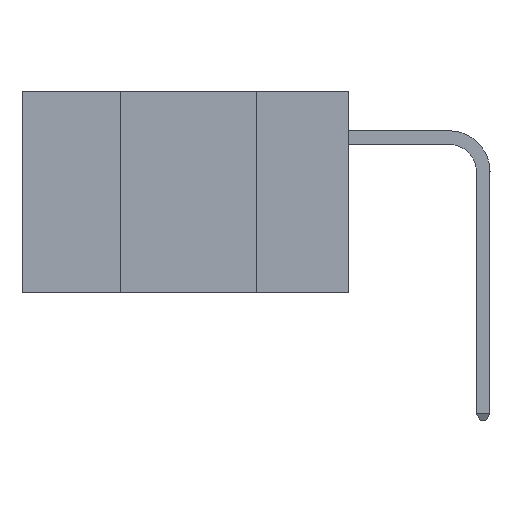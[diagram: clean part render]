
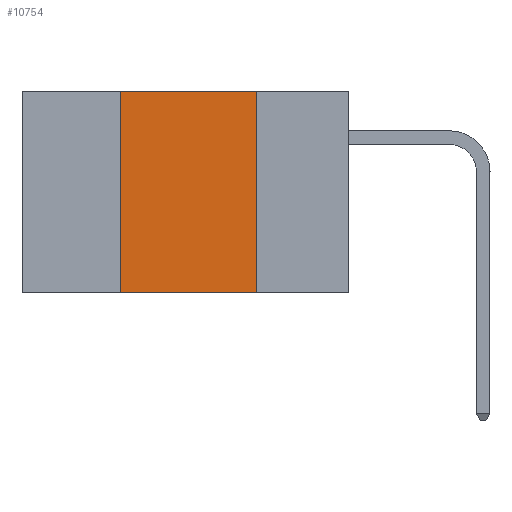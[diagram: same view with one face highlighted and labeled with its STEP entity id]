
A CAD part, left-side view. The second image highlights one B-rep face of the part: STEP entity #10754.
In plain terms, the highlighted planar face has unit normal (-1, 0, 0).
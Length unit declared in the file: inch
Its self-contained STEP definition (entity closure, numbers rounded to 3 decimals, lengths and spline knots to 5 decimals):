
#1278 = LINE ( 'NONE', #29180, #15102 ) ;
#1377 = AXIS2_PLACEMENT_3D ( 'NONE', #20924, #40406, #5973 ) ;
#1792 = EDGE_CURVE ( 'NONE', #21485, #6824, #11633, .T. ) ;
#2624 = DIRECTION ( 'NONE',  ( 0., 0., -1. ) ) ;
#2697 = EDGE_CURVE ( 'NONE', #21485, #25090, #6118, .T. ) ;
#4278 = LINE ( 'NONE', #31391, #24655 ) ;
#5049 = ORIENTED_EDGE ( 'NONE', *, *, #48254, .F. ) ;
#5973 = DIRECTION ( 'NONE',  ( 0., 0., -1. ) ) ;
#6118 = LINE ( 'NONE', #34220, #27786 ) ;
#6824 = VERTEX_POINT ( 'NONE', #37957 ) ;
#10754 = ADVANCED_FACE ( 'NONE', ( #14118 ), #32382, .F. ) ;
#11633 = LINE ( 'NONE', #17485, #30293 ) ;
#12376 = EDGE_CURVE ( 'NONE', #15441, #6824, #1278, .T. ) ;
#13359 = DIRECTION ( 'NONE',  ( 0., -1., 0. ) ) ;
#13405 = CARTESIAN_POINT ( 'NONE',  ( 0., 0.42, 0. ) ) ;
#13612 = DIRECTION ( 'NONE',  ( 0., -1., 0. ) ) ;
#14118 = FACE_OUTER_BOUND ( 'NONE', #40738, .T. ) ;
#15102 = VECTOR ( 'NONE', #2624, 39.37008 ) ;
#15112 = ORIENTED_EDGE ( 'NONE', *, *, #1792, .T. ) ;
#15441 = VERTEX_POINT ( 'NONE', #28796 ) ;
#16535 = ORIENTED_EDGE ( 'NONE', *, *, #12376, .F. ) ;
#17485 = CARTESIAN_POINT ( 'NONE',  ( 0., 0.6, -0.37 ) ) ;
#20924 = CARTESIAN_POINT ( 'NONE',  ( 0., 0.6, 0. ) ) ;
#21485 = VERTEX_POINT ( 'NONE', #27293 ) ;
#22627 = DIRECTION ( 'NONE',  ( 0., 0., 1. ) ) ;
#24655 = VECTOR ( 'NONE', #13359, 39.37008 ) ;
#25090 = VERTEX_POINT ( 'NONE', #13405 ) ;
#27293 = CARTESIAN_POINT ( 'NONE',  ( 0., 0.42, -0.37 ) ) ;
#27786 = VECTOR ( 'NONE', #22627, 39.37008 ) ;
#28721 = ORIENTED_EDGE ( 'NONE', *, *, #2697, .F. ) ;
#28796 = CARTESIAN_POINT ( 'NONE',  ( 0., 0.17, 0. ) ) ;
#29180 = CARTESIAN_POINT ( 'NONE',  ( 0., 0.17, 0. ) ) ;
#30293 = VECTOR ( 'NONE', #13612, 39.37008 ) ;
#31391 = CARTESIAN_POINT ( 'NONE',  ( 0., 0.6, 0. ) ) ;
#32382 = PLANE ( 'NONE',  #1377 ) ;
#34220 = CARTESIAN_POINT ( 'NONE',  ( 0., 0.42, 0. ) ) ;
#37957 = CARTESIAN_POINT ( 'NONE',  ( 0., 0.17, -0.37 ) ) ;
#40406 = DIRECTION ( 'NONE',  ( 1., 0., 0. ) ) ;
#40738 = EDGE_LOOP ( 'NONE', ( #16535, #5049, #28721, #15112 ) ) ;
#48254 = EDGE_CURVE ( 'NONE', #25090, #15441, #4278, .T. ) ;
